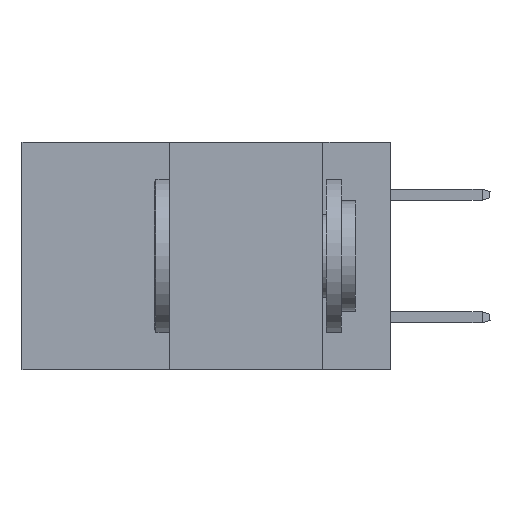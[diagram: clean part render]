
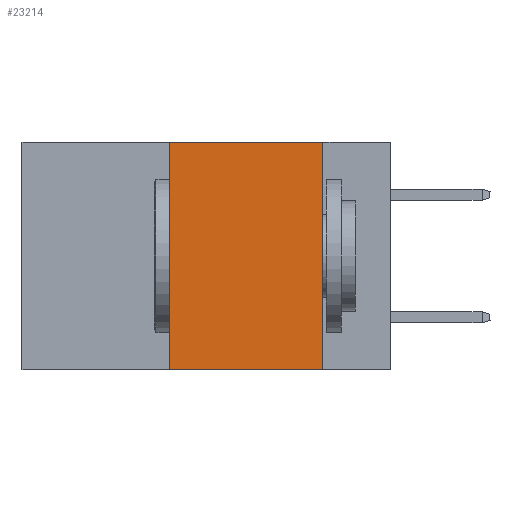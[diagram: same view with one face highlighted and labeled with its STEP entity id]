
A CAD part, left-side view. The second image highlights one B-rep face of the part: STEP entity #23214.
In plain terms, the highlighted planar face has unit normal (-1, 0, 0).
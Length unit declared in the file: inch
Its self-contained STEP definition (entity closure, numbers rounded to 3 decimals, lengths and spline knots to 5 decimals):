
#1239 = ORIENTED_EDGE ( 'NONE', *, *, #15650, .F. ) ;
#1244 = EDGE_CURVE ( 'NONE', #15763, #21446, #10699, .T. ) ;
#1273 = LINE ( 'NONE', #6705, #11246 ) ;
#1364 = EDGE_CURVE ( 'NONE', #21446, #13849, #7894, .T. ) ;
#2011 = CARTESIAN_POINT ( 'NONE',  ( 0., 0.36, 0. ) ) ;
#2773 = VECTOR ( 'NONE', #17680, 39.37008 ) ;
#3062 = ORIENTED_EDGE ( 'NONE', *, *, #14977, .T. ) ;
#3100 = CARTESIAN_POINT ( 'NONE',  ( 0., 0.6, 0. ) ) ;
#3618 = PLANE ( 'NONE',  #23302 ) ;
#4675 = DIRECTION ( 'NONE',  ( 0., 0., 1. ) ) ;
#5397 = CARTESIAN_POINT ( 'NONE',  ( 0., 0.36, -0.37 ) ) ;
#5545 = DIRECTION ( 'NONE',  ( 1., 0., 0. ) ) ;
#6007 = CARTESIAN_POINT ( 'NONE',  ( 0., 0.36, 0. ) ) ;
#6070 = LINE ( 'NONE', #14160, #15079 ) ;
#6264 = FACE_OUTER_BOUND ( 'NONE', #17740, .T. ) ;
#6705 = CARTESIAN_POINT ( 'NONE',  ( 0., 0.6, -0.37 ) ) ;
#7011 = DIRECTION ( 'NONE',  ( 0., 0., -1. ) ) ;
#7894 = LINE ( 'NONE', #3100, #2773 ) ;
#9166 = VERTEX_POINT ( 'NONE', #19141 ) ;
#9172 = CARTESIAN_POINT ( 'NONE',  ( 0., 0.6, 0. ) ) ;
#9397 = CARTESIAN_POINT ( 'NONE',  ( 0., 0.11, 0. ) ) ;
#10699 = LINE ( 'NONE', #6007, #18915 ) ;
#11246 = VECTOR ( 'NONE', #19094, 39.37008 ) ;
#11780 = ORIENTED_EDGE ( 'NONE', *, *, #1364, .F. ) ;
#13849 = VERTEX_POINT ( 'NONE', #9397 ) ;
#14160 = CARTESIAN_POINT ( 'NONE',  ( 0., 0.11, 0. ) ) ;
#14977 = EDGE_CURVE ( 'NONE', #15763, #9166, #1273, .T. ) ;
#15079 = VECTOR ( 'NONE', #7011, 39.37008 ) ;
#15650 = EDGE_CURVE ( 'NONE', #13849, #9166, #6070, .T. ) ;
#15763 = VERTEX_POINT ( 'NONE', #5397 ) ;
#16980 = ORIENTED_EDGE ( 'NONE', *, *, #1244, .F. ) ;
#17680 = DIRECTION ( 'NONE',  ( 0., -1., 0. ) ) ;
#17740 = EDGE_LOOP ( 'NONE', ( #1239, #11780, #16980, #3062 ) ) ;
#18043 = DIRECTION ( 'NONE',  ( 0., 0., -1. ) ) ;
#18915 = VECTOR ( 'NONE', #4675, 39.37008 ) ;
#19094 = DIRECTION ( 'NONE',  ( 0., -1., 0. ) ) ;
#19141 = CARTESIAN_POINT ( 'NONE',  ( 0., 0.11, -0.37 ) ) ;
#21446 = VERTEX_POINT ( 'NONE', #2011 ) ;
#23214 = ADVANCED_FACE ( 'NONE', ( #6264 ), #3618, .F. ) ;
#23302 = AXIS2_PLACEMENT_3D ( 'NONE', #9172, #5545, #18043 ) ;
